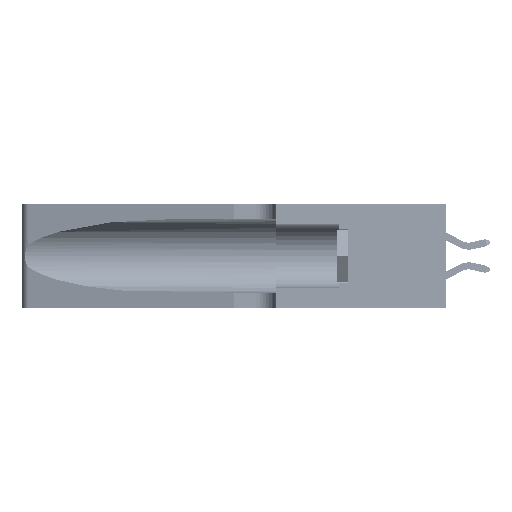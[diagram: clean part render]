
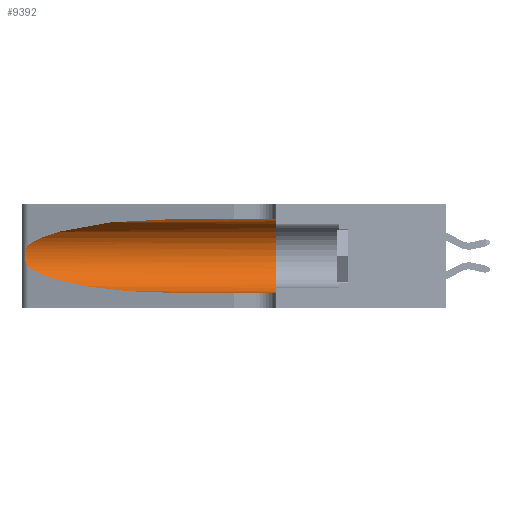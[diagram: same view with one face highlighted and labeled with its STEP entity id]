
A CAD part, left-side view. The second image highlights one B-rep face of the part: STEP entity #9392.
In plain terms, the highlighted cylindrical face has radius 3.308 mm (diameter 6.617 mm), a partial arc.
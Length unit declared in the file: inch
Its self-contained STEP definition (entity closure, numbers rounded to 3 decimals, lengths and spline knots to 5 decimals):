
#1370 = CARTESIAN_POINT ( 'NONE',  ( 0.25789, 1.23486, 0.15765 ) ) ;
#1526 = CARTESIAN_POINT ( 'NONE',  ( 0.25487, 1.22718, 0.14631 ) ) ;
#2519 = LINE ( 'NONE', #21075, #29211 ) ;
#3134 = CARTESIAN_POINT ( 'NONE',  ( 0.25487, 1.22718, 0.14631 ) ) ;
#3150 = EDGE_CURVE ( 'NONE', #39131, #3471, #42614, .T. ) ;
#3471 = VERTEX_POINT ( 'NONE', #43332 ) ;
#3496 = FACE_OUTER_BOUND ( 'NONE', #23284, .T. ) ;
#4434 = ORIENTED_EDGE ( 'NONE', *, *, #9728, .T. ) ;
#4738 = CARTESIAN_POINT ( 'NONE',  ( 0.25555, 1.22993, 0.14849 ) ) ;
#5624 = ORIENTED_EDGE ( 'NONE', *, *, #43397, .T. ) ;
#5844 =( BOUNDED_CURVE ( )  B_SPLINE_CURVE ( 3, ( #12906, #44152, #41091, #20132 ),
 .UNSPECIFIED., .F., .F. ) 
 B_SPLINE_CURVE_WITH_KNOTS ( ( 4, 4 ),
 ( 1.5708, 2.84003 ),
 .UNSPECIFIED. ) 
 CURVE ( )  GEOMETRIC_REPRESENTATION_ITEM ( )  RATIONAL_B_SPLINE_CURVE ( ( 1., 0.87, 0.87, 1. ) ) 
 REPRESENTATION_ITEM ( '' )  );
#6053 = VERTEX_POINT ( 'NONE', #42841 ) ;
#6611 = EDGE_CURVE ( 'NONE', #6053, #8074, #17323, .T. ) ;
#6653 = CARTESIAN_POINT ( 'NONE',  ( 0.1305, 0.35, 0.185 ) ) ;
#6899 = VERTEX_POINT ( 'NONE', #24661 ) ;
#7266 = DIRECTION ( 'NONE',  ( 0., 0., -1. ) ) ;
#8069 = CARTESIAN_POINT ( 'NONE',  ( 0.25639, 1.23186, 0.15144 ) ) ;
#8074 = VERTEX_POINT ( 'NONE', #3134 ) ;
#8182 = CARTESIAN_POINT ( 'NONE',  ( 0.18966, 0.96281, 0.05475 ) ) ;
#8707 = CARTESIAN_POINT ( 'NONE',  ( 0.1305, 0.35, 0.31525 ) ) ;
#9392 = ADVANCED_FACE ( 'NONE', ( #3496 ), #15481, .F. ) ;
#9728 = EDGE_CURVE ( 'NONE', #8074, #6899, #20953, .T. ) ;
#10469 = CARTESIAN_POINT ( 'NONE',  ( 0.1305, 1.61858, 0.185 ) ) ;
#10856 = EDGE_CURVE ( 'NONE', #33139, #39131, #2519, .T. ) ;
#12214 = AXIS2_PLACEMENT_3D ( 'NONE', #10469, #27995, #7266 ) ;
#12906 = CARTESIAN_POINT ( 'NONE',  ( 0.1305, 0.72297, 0.31525 ) ) ;
#13127 = ORIENTED_EDGE ( 'NONE', *, *, #32112, .T. ) ;
#15316 = CARTESIAN_POINT ( 'NONE',  ( 0.25487, 1.22718, 0.14631 ) ) ;
#15481 = CYLINDRICAL_SURFACE ( 'NONE', #12214, 0.13025 ) ;
#17323 = B_SPLINE_CURVE_WITH_KNOTS ( 'NONE', 3,
 ( #25598, #39438, #18897, #25737, #32873, #28934, #43085, #25878, #43393, #32432, #1370, #8069, #4738, #1526 ),
 .UNSPECIFIED., .F., .F.,
 ( 4, 2, 2, 2, 2, 2, 4 ),
 ( 0., 0.00027, 0.00053, 0.00107, 0.0016, 0.00187, 0.00214 ),
 .UNSPECIFIED. ) ;
#18785 = CARTESIAN_POINT ( 'NONE',  ( 0.1305, 1.61858, 0.05475 ) ) ;
#18897 = CARTESIAN_POINT ( 'NONE',  ( 0.25639, 1.23184, 0.21858 ) ) ;
#19157 = CARTESIAN_POINT ( 'NONE',  ( 0.2373, 1.15595, 0.08982 ) ) ;
#20132 = CARTESIAN_POINT ( 'NONE',  ( 0.25487, 1.22718, 0.22369 ) ) ;
#20953 =( BOUNDED_CURVE ( )  B_SPLINE_CURVE ( 3, ( #15316, #19157, #8182, #39974 ),
 .UNSPECIFIED., .F., .F. ) 
 B_SPLINE_CURVE_WITH_KNOTS ( ( 4, 4 ),
 ( 3.44316, 4.71239 ),
 .UNSPECIFIED. ) 
 CURVE ( )  GEOMETRIC_REPRESENTATION_ITEM ( )  RATIONAL_B_SPLINE_CURVE ( ( 1., 0.87, 0.87, 1. ) ) 
 REPRESENTATION_ITEM ( '' )  );
#21075 = CARTESIAN_POINT ( 'NONE',  ( 0.1305, 1.61858, 0.31525 ) ) ;
#21817 = DIRECTION ( 'NONE',  ( 0., -1., 0. ) ) ;
#22650 = ORIENTED_EDGE ( 'NONE', *, *, #3150, .F. ) ;
#23284 = EDGE_LOOP ( 'NONE', ( #5624, #23527, #4434, #13127, #22650, #25573 ) ) ;
#23527 = ORIENTED_EDGE ( 'NONE', *, *, #6611, .T. ) ;
#24317 = CARTESIAN_POINT ( 'NONE',  ( 0.1305, 0.72297, 0.31525 ) ) ;
#24661 = CARTESIAN_POINT ( 'NONE',  ( 0.1305, 0.72297, 0.05475 ) ) ;
#25573 = ORIENTED_EDGE ( 'NONE', *, *, #10856, .F. ) ;
#25598 = CARTESIAN_POINT ( 'NONE',  ( 0.25487, 1.22718, 0.22369 ) ) ;
#25737 = CARTESIAN_POINT ( 'NONE',  ( 0.25787, 1.23484, 0.2124 ) ) ;
#25878 = CARTESIAN_POINT ( 'NONE',  ( 0.26075, 1.23896, 0.178 ) ) ;
#27995 = DIRECTION ( 'NONE',  ( 0., -1., 0. ) ) ;
#28661 = DIRECTION ( 'NONE',  ( 0., -1., 0. ) ) ;
#28797 = VECTOR ( 'NONE', #28661, 39.37008 ) ;
#28934 = CARTESIAN_POINT ( 'NONE',  ( 0.26018, 1.23835, 0.19895 ) ) ;
#29211 = VECTOR ( 'NONE', #21817, 39.37008 ) ;
#31977 = LINE ( 'NONE', #18785, #28797 ) ;
#32112 = EDGE_CURVE ( 'NONE', #6899, #3471, #31977, .T. ) ;
#32432 = CARTESIAN_POINT ( 'NONE',  ( 0.25856, 1.23593, 0.16098 ) ) ;
#32873 = CARTESIAN_POINT ( 'NONE',  ( 0.25854, 1.2359, 0.20912 ) ) ;
#33139 = VERTEX_POINT ( 'NONE', #24317 ) ;
#34247 = DIRECTION ( 'NONE',  ( 0., 0., 1. ) ) ;
#39131 = VERTEX_POINT ( 'NONE', #8707 ) ;
#39438 = CARTESIAN_POINT ( 'NONE',  ( 0.25555, 1.22994, 0.2215 ) ) ;
#39974 = CARTESIAN_POINT ( 'NONE',  ( 0.1305, 0.72297, 0.05475 ) ) ;
#41072 = DIRECTION ( 'NONE',  ( 0., 1., 0. ) ) ;
#41091 = CARTESIAN_POINT ( 'NONE',  ( 0.2373, 1.15595, 0.28018 ) ) ;
#42614 = CIRCLE ( 'NONE', #44525, 0.13025 ) ;
#42841 = CARTESIAN_POINT ( 'NONE',  ( 0.25487, 1.22718, 0.22369 ) ) ;
#43085 = CARTESIAN_POINT ( 'NONE',  ( 0.26075, 1.23896, 0.19203 ) ) ;
#43332 = CARTESIAN_POINT ( 'NONE',  ( 0.1305, 0.35, 0.05475 ) ) ;
#43393 = CARTESIAN_POINT ( 'NONE',  ( 0.26017, 1.23833, 0.17102 ) ) ;
#43397 = EDGE_CURVE ( 'NONE', #33139, #6053, #5844, .T. ) ;
#44152 = CARTESIAN_POINT ( 'NONE',  ( 0.18966, 0.96281, 0.31525 ) ) ;
#44525 = AXIS2_PLACEMENT_3D ( 'NONE', #6653, #41072, #34247 ) ;
